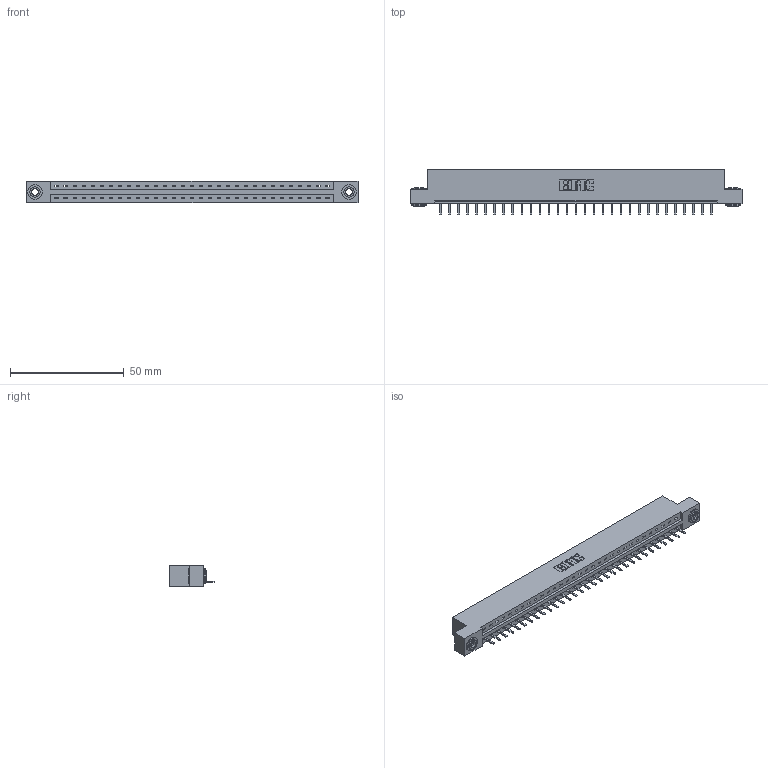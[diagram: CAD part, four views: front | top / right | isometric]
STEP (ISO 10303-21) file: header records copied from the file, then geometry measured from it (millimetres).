
FILE_DESCRIPTION (( 'STEP AP203' ), '1' );
FILE_NAME ('337-031-520-103.STEP', '2018-08-07T02:51:40', ( '' ), ( '' ), 'SwSTEP 2.0', 'SolidWorks 2016', '' );
FILE_SCHEMA (( 'CONFIG_CONTROL_DESIGN' ));
Length unit declared in the file: inch
Products named in the file (4): 337 Part_Flush Mounting Lugs - 0.156 Dia-TH; 345-292-001_345-293-120; 345-250-002_345-250-002-102; 337-031-520-103
Assembly tree (34 placements, depth 2):
  337-031-520-103
    337 Part_Flush Mounting Lugs - 0.156 Dia-TH
    345-292-001_345-293-120  x31
    345-250-002_345-250-002-102  x2
Bounding box: 145.85 x 20.02 x 9.4 mm (x, y, z)
Volume: 14950.9 mm3; surface area: 15300.2 mm2
Topology: 34 solids, 34 shells, 2198 faces, 6463 edges, 4222 vertices
Faces by surface type: plane 1568, cylinder 622, cone 8
Entity records: 25230 total; most frequent: CARTESIAN_POINT 4382, ORIENTED_EDGE 4330, DIRECTION 3733, EDGE_CURVE 2165, LINE 2009, VECTOR 2009, VERTEX_POINT 1438, AXIS2_PLACEMENT_3D 862
